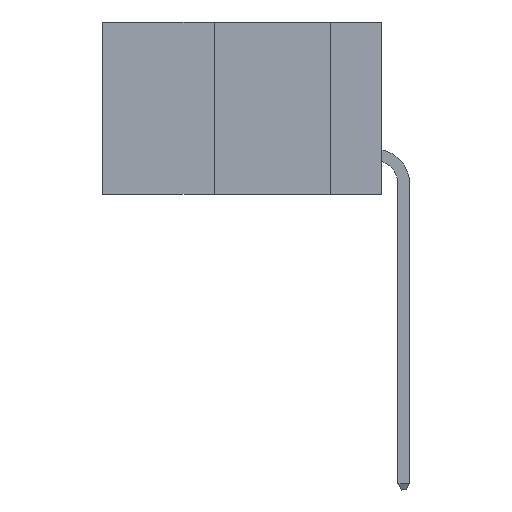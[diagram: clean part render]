
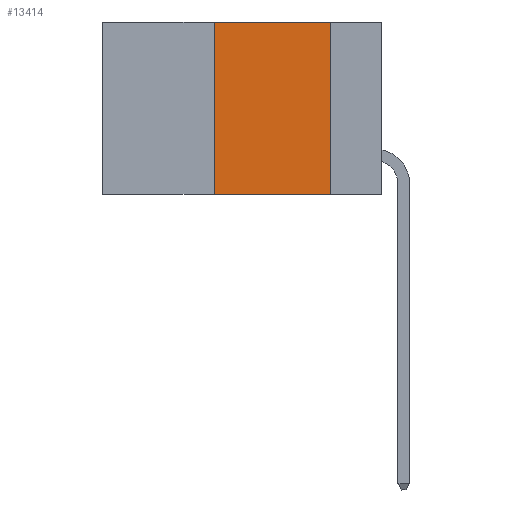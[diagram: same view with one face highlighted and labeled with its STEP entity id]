
A CAD part, left-side view. The second image highlights one B-rep face of the part: STEP entity #13414.
In plain terms, the highlighted planar face has unit normal (-1, 0, 0).
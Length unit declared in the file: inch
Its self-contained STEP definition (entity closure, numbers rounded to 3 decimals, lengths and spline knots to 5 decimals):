
#1414 = LINE ( 'NONE', #6291, #15661 ) ;
#1465 = LINE ( 'NONE', #9539, #6505 ) ;
#3771 = FACE_OUTER_BOUND ( 'NONE', #20906, .T. ) ;
#4378 = CARTESIAN_POINT ( 'NONE',  ( 0., 0.36, -0.37 ) ) ;
#5844 = ORIENTED_EDGE ( 'NONE', *, *, #12222, .F. ) ;
#5860 = PLANE ( 'NONE',  #8199 ) ;
#6291 = CARTESIAN_POINT ( 'NONE',  ( 0., 0.11, 0. ) ) ;
#6505 = VECTOR ( 'NONE', #22203, 39.37008 ) ;
#6881 = CARTESIAN_POINT ( 'NONE',  ( 0., 0.11, 0. ) ) ;
#7762 = DIRECTION ( 'NONE',  ( 1., 0., 0. ) ) ;
#8085 = EDGE_CURVE ( 'NONE', #20198, #17621, #8342, .T. ) ;
#8199 = AXIS2_PLACEMENT_3D ( 'NONE', #13290, #7762, #20535 ) ;
#8274 = DIRECTION ( 'NONE',  ( 0., -1., 0. ) ) ;
#8342 = LINE ( 'NONE', #17379, #9509 ) ;
#9347 = EDGE_CURVE ( 'NONE', #20198, #12088, #16970, .T. ) ;
#9509 = VECTOR ( 'NONE', #8274, 39.37008 ) ;
#9539 = CARTESIAN_POINT ( 'NONE',  ( 0., 0.6, 0. ) ) ;
#9747 = CARTESIAN_POINT ( 'NONE',  ( 0., 0.11, -0.37 ) ) ;
#9939 = CARTESIAN_POINT ( 'NONE',  ( 0., 0.36, 0. ) ) ;
#10881 = ORIENTED_EDGE ( 'NONE', *, *, #9347, .F. ) ;
#12088 = VERTEX_POINT ( 'NONE', #20033 ) ;
#12189 = VECTOR ( 'NONE', #13615, 39.37008 ) ;
#12222 = EDGE_CURVE ( 'NONE', #12088, #21063, #1465, .T. ) ;
#13056 = EDGE_CURVE ( 'NONE', #21063, #17621, #1414, .T. ) ;
#13290 = CARTESIAN_POINT ( 'NONE',  ( 0., 0.6, 0. ) ) ;
#13414 = ADVANCED_FACE ( 'NONE', ( #3771 ), #5860, .F. ) ;
#13615 = DIRECTION ( 'NONE',  ( 0., 0., 1. ) ) ;
#15462 = DIRECTION ( 'NONE',  ( 0., 0., -1. ) ) ;
#15661 = VECTOR ( 'NONE', #15462, 39.37008 ) ;
#16970 = LINE ( 'NONE', #9939, #12189 ) ;
#17379 = CARTESIAN_POINT ( 'NONE',  ( 0., 0.6, -0.37 ) ) ;
#17621 = VERTEX_POINT ( 'NONE', #9747 ) ;
#19361 = ORIENTED_EDGE ( 'NONE', *, *, #13056, .F. ) ;
#20033 = CARTESIAN_POINT ( 'NONE',  ( 0., 0.36, 0. ) ) ;
#20198 = VERTEX_POINT ( 'NONE', #4378 ) ;
#20481 = ORIENTED_EDGE ( 'NONE', *, *, #8085, .T. ) ;
#20535 = DIRECTION ( 'NONE',  ( 0., 0., -1. ) ) ;
#20906 = EDGE_LOOP ( 'NONE', ( #19361, #5844, #10881, #20481 ) ) ;
#21063 = VERTEX_POINT ( 'NONE', #6881 ) ;
#22203 = DIRECTION ( 'NONE',  ( 0., -1., 0. ) ) ;
